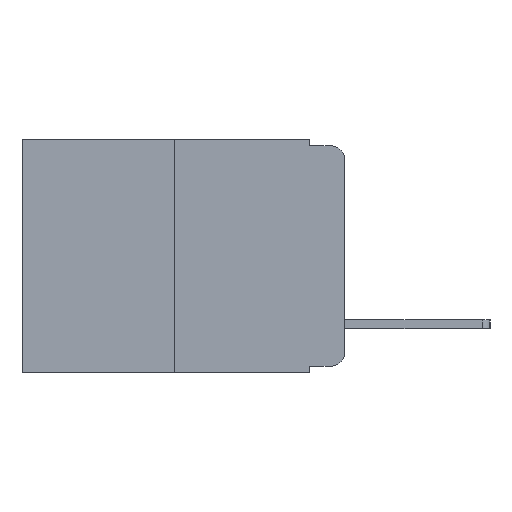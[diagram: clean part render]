
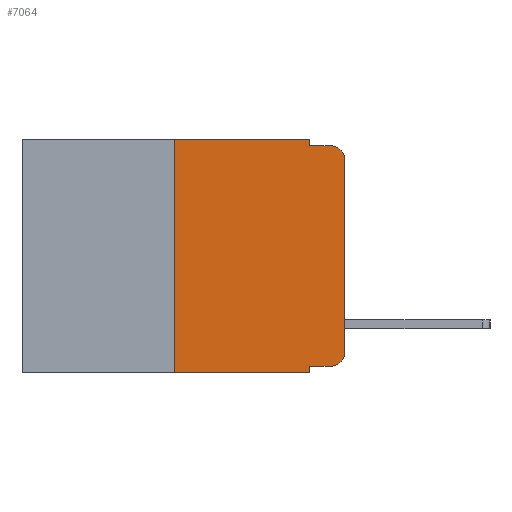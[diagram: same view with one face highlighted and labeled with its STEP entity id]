
A CAD part, left-side view. The second image highlights one B-rep face of the part: STEP entity #7064.
In plain terms, the highlighted planar face has unit normal (-1, 0, 0).
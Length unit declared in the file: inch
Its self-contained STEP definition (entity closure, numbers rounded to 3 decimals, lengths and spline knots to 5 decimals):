
#175 = DIRECTION ( 'NONE',  ( 0., -1., 0. ) ) ;
#413 = ORIENTED_EDGE ( 'NONE', *, *, #8734, .F. ) ;
#581 = EDGE_CURVE ( 'NONE', #7643, #13558, #10728, .T. ) ;
#613 = VERTEX_POINT ( 'NONE', #7143 ) ;
#704 = DIRECTION ( 'NONE',  ( 0., 0., -1. ) ) ;
#831 = VERTEX_POINT ( 'NONE', #9492 ) ;
#1084 = LINE ( 'NONE', #9408, #17127 ) ;
#1248 = ORIENTED_EDGE ( 'NONE', *, *, #19570, .T. ) ;
#1384 = CARTESIAN_POINT ( 'NONE',  ( 0., 0.051, 0. ) ) ;
#2094 = CARTESIAN_POINT ( 'NONE',  ( 0., 0.051, 0. ) ) ;
#2140 = CARTESIAN_POINT ( 'NONE',  ( 0., 0.051, -0.01 ) ) ;
#2364 = LINE ( 'NONE', #2140, #14368 ) ;
#2411 = VECTOR ( 'NONE', #18249, 39.37008 ) ;
#3007 = CARTESIAN_POINT ( 'NONE',  ( 0., 0., 0. ) ) ;
#3041 = LINE ( 'NONE', #6955, #14522 ) ;
#3050 = DIRECTION ( 'NONE',  ( 0., 0., -1. ) ) ;
#3302 = DIRECTION ( 'NONE',  ( 0., -1., 0. ) ) ;
#3305 = VERTEX_POINT ( 'NONE', #17657 ) ;
#4315 = VECTOR ( 'NONE', #3050, 39.37008 ) ;
#4426 = EDGE_CURVE ( 'NONE', #831, #3305, #3041, .T. ) ;
#4502 = CARTESIAN_POINT ( 'NONE',  ( 0., 0.02, -0.03 ) ) ;
#4504 = CARTESIAN_POINT ( 'NONE',  ( 0., 0.051, -0.01 ) ) ;
#4824 = ORIENTED_EDGE ( 'NONE', *, *, #13689, .F. ) ;
#5528 = DIRECTION ( 'NONE',  ( -1., 0., 0. ) ) ;
#5639 = EDGE_CURVE ( 'NONE', #8112, #16752, #11570, .T. ) ;
#5727 = CARTESIAN_POINT ( 'NONE',  ( 0., 0.02, -0.313 ) ) ;
#5797 = VECTOR ( 'NONE', #3302, 39.37008 ) ;
#6047 = ORIENTED_EDGE ( 'NONE', *, *, #8480, .F. ) ;
#6079 = DIRECTION ( 'NONE',  ( 0., 0., -1. ) ) ;
#6282 = ORIENTED_EDGE ( 'NONE', *, *, #10867, .F. ) ;
#6955 = CARTESIAN_POINT ( 'NONE',  ( 0., 0.473, -0.343 ) ) ;
#7064 = ADVANCED_FACE ( 'NONE', ( #11751 ), #19185, .F. ) ;
#7099 = CARTESIAN_POINT ( 'NONE',  ( 0., 0.02, -0.333 ) ) ;
#7118 = CARTESIAN_POINT ( 'NONE',  ( 0., 0.473, 0. ) ) ;
#7134 = AXIS2_PLACEMENT_3D ( 'NONE', #5727, #5528, #13729 ) ;
#7143 = CARTESIAN_POINT ( 'NONE',  ( 0., 0.02, -0.01 ) ) ;
#7228 = CARTESIAN_POINT ( 'NONE',  ( 0., 0.051, 0. ) ) ;
#7643 = VERTEX_POINT ( 'NONE', #7099 ) ;
#8042 = VERTEX_POINT ( 'NONE', #11069 ) ;
#8112 = VERTEX_POINT ( 'NONE', #2094 ) ;
#8124 = VERTEX_POINT ( 'NONE', #19021 ) ;
#8480 = EDGE_CURVE ( 'NONE', #831, #8124, #1084, .T. ) ;
#8734 = EDGE_CURVE ( 'NONE', #16752, #613, #2364, .T. ) ;
#9240 = DIRECTION ( 'NONE',  ( 0., -1., 0. ) ) ;
#9408 = CARTESIAN_POINT ( 'NONE',  ( 0., 0.25, 0. ) ) ;
#9492 = CARTESIAN_POINT ( 'NONE',  ( 0., 0.25, -0.343 ) ) ;
#9777 = EDGE_CURVE ( 'NONE', #10141, #613, #17289, .T. ) ;
#10141 = VERTEX_POINT ( 'NONE', #17643 ) ;
#10223 = DIRECTION ( 'NONE',  ( 1., 0., 0. ) ) ;
#10403 = ORIENTED_EDGE ( 'NONE', *, *, #9777, .T. ) ;
#10658 = ORIENTED_EDGE ( 'NONE', *, *, #4426, .T. ) ;
#10728 = CIRCLE ( 'NONE', #7134, 0.02 ) ;
#10867 = EDGE_CURVE ( 'NONE', #8124, #8112, #14512, .T. ) ;
#11069 = CARTESIAN_POINT ( 'NONE',  ( 0., 0.051, -0.333 ) ) ;
#11266 = LINE ( 'NONE', #3007, #2411 ) ;
#11570 = LINE ( 'NONE', #7228, #14236 ) ;
#11751 = FACE_OUTER_BOUND ( 'NONE', #13996, .T. ) ;
#11760 = VECTOR ( 'NONE', #9240, 39.37008 ) ;
#12024 = CARTESIAN_POINT ( 'NONE',  ( 0., 0., -0.313 ) ) ;
#12356 = CARTESIAN_POINT ( 'NONE',  ( 0., 0.051, -0.333 ) ) ;
#12523 = DIRECTION ( 'NONE',  ( 0., 0., 1. ) ) ;
#12570 = LINE ( 'NONE', #1384, #4315 ) ;
#12770 = AXIS2_PLACEMENT_3D ( 'NONE', #7118, #10223, #704 ) ;
#13558 = VERTEX_POINT ( 'NONE', #12024 ) ;
#13564 = ORIENTED_EDGE ( 'NONE', *, *, #18853, .T. ) ;
#13689 = EDGE_CURVE ( 'NONE', #8042, #3305, #12570, .T. ) ;
#13729 = DIRECTION ( 'NONE',  ( 0., 0., -1. ) ) ;
#13996 = EDGE_LOOP ( 'NONE', ( #13564, #10403, #413, #19286, #6282, #6047, #10658, #4824, #1248, #14071 ) ) ;
#14071 = ORIENTED_EDGE ( 'NONE', *, *, #581, .T. ) ;
#14236 = VECTOR ( 'NONE', #15420, 39.37008 ) ;
#14368 = VECTOR ( 'NONE', #17608, 39.37008 ) ;
#14491 = AXIS2_PLACEMENT_3D ( 'NONE', #4502, #15319, #6079 ) ;
#14512 = LINE ( 'NONE', #18566, #5797 ) ;
#14522 = VECTOR ( 'NONE', #175, 39.37008 ) ;
#15319 = DIRECTION ( 'NONE',  ( -1., 0., 0. ) ) ;
#15420 = DIRECTION ( 'NONE',  ( 0., 0., -1. ) ) ;
#15809 = LINE ( 'NONE', #12356, #11760 ) ;
#16752 = VERTEX_POINT ( 'NONE', #4504 ) ;
#17127 = VECTOR ( 'NONE', #12523, 39.37008 ) ;
#17289 = CIRCLE ( 'NONE', #14491, 0.02 ) ;
#17608 = DIRECTION ( 'NONE',  ( 0., -1., 0. ) ) ;
#17643 = CARTESIAN_POINT ( 'NONE',  ( 0., 0., -0.03 ) ) ;
#17657 = CARTESIAN_POINT ( 'NONE',  ( 0., 0.051, -0.343 ) ) ;
#18249 = DIRECTION ( 'NONE',  ( 0., 0., 1. ) ) ;
#18566 = CARTESIAN_POINT ( 'NONE',  ( 0., 0.473, 0. ) ) ;
#18853 = EDGE_CURVE ( 'NONE', #13558, #10141, #11266, .T. ) ;
#19021 = CARTESIAN_POINT ( 'NONE',  ( 0., 0.25, 0. ) ) ;
#19185 = PLANE ( 'NONE',  #12770 ) ;
#19286 = ORIENTED_EDGE ( 'NONE', *, *, #5639, .F. ) ;
#19570 = EDGE_CURVE ( 'NONE', #8042, #7643, #15809, .T. ) ;
